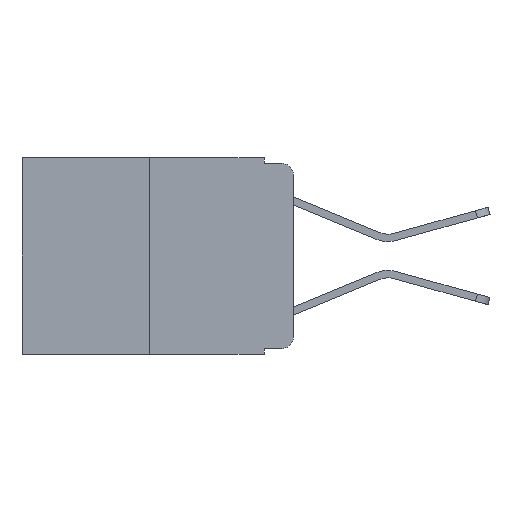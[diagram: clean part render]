
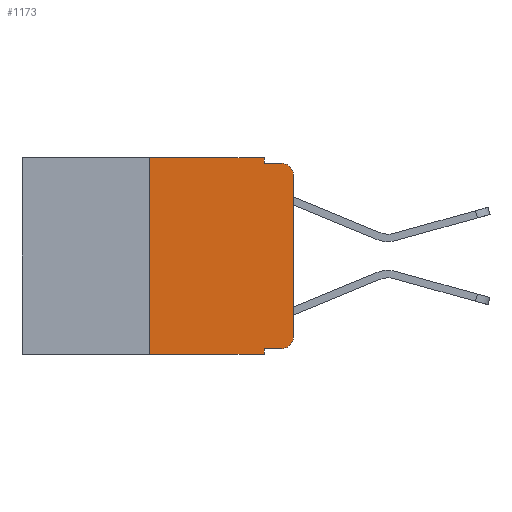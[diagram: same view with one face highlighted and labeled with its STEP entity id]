
A CAD part, left-side view. The second image highlights one B-rep face of the part: STEP entity #1173.
In plain terms, the highlighted planar face has unit normal (-1, 0, 0).
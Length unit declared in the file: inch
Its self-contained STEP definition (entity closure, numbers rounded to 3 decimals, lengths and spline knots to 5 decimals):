
#42 = DIRECTION ( 'NONE',  ( -1., 0., 0. ) ) ;
#172 = VERTEX_POINT ( 'NONE', #10972 ) ;
#308 = DIRECTION ( 'NONE',  ( 0., -1., 0. ) ) ;
#426 = EDGE_CURVE ( 'NONE', #25586, #172, #12682, .T. ) ;
#539 = CARTESIAN_POINT ( 'NONE',  ( 0., 0., -0.313 ) ) ;
#889 = DIRECTION ( 'NONE',  ( 0., 0., 1. ) ) ;
#1173 = ADVANCED_FACE ( 'NONE', ( #11707 ), #22429, .F. ) ;
#1583 = VECTOR ( 'NONE', #889, 39.37008 ) ;
#1644 = CARTESIAN_POINT ( 'NONE',  ( 0., 0.051, -0.333 ) ) ;
#1683 = VECTOR ( 'NONE', #18748, 39.37008 ) ;
#1725 = DIRECTION ( 'NONE',  ( 0., -1., 0. ) ) ;
#1880 = EDGE_CURVE ( 'NONE', #25586, #25574, #18023, .T. ) ;
#1989 = ORIENTED_EDGE ( 'NONE', *, *, #12848, .T. ) ;
#2094 = VECTOR ( 'NONE', #1725, 39.37008 ) ;
#2665 = VERTEX_POINT ( 'NONE', #5223 ) ;
#3000 = CARTESIAN_POINT ( 'NONE',  ( 0., 0.02, -0.313 ) ) ;
#3271 = EDGE_CURVE ( 'NONE', #6825, #2665, #11036, .T. ) ;
#3290 = ORIENTED_EDGE ( 'NONE', *, *, #10159, .F. ) ;
#5088 = DIRECTION ( 'NONE',  ( 0., 0., -1. ) ) ;
#5223 = CARTESIAN_POINT ( 'NONE',  ( 0., 0.25, 0. ) ) ;
#6825 = VERTEX_POINT ( 'NONE', #17806 ) ;
#7076 = VECTOR ( 'NONE', #25729, 39.37008 ) ;
#7165 = CARTESIAN_POINT ( 'NONE',  ( 0., 0.473, 0. ) ) ;
#7501 = CIRCLE ( 'NONE', #18302, 0.02 ) ;
#8603 = CARTESIAN_POINT ( 'NONE',  ( 0., 0., -0.03 ) ) ;
#8751 = ORIENTED_EDGE ( 'NONE', *, *, #16647, .F. ) ;
#9027 = VERTEX_POINT ( 'NONE', #9641 ) ;
#9124 = CARTESIAN_POINT ( 'NONE',  ( 0., 0.25, 0. ) ) ;
#9384 = EDGE_LOOP ( 'NONE', ( #11622, #1989, #24261, #3290, #8751, #14780, #20211, #15404, #26097, #10689 ) ) ;
#9475 = VECTOR ( 'NONE', #15234, 39.37008 ) ;
#9641 = CARTESIAN_POINT ( 'NONE',  ( 0., 0.051, 0. ) ) ;
#10159 = EDGE_CURVE ( 'NONE', #9027, #24816, #17827, .T. ) ;
#10689 = ORIENTED_EDGE ( 'NONE', *, *, #24200, .T. ) ;
#10972 = CARTESIAN_POINT ( 'NONE',  ( 0., 0.02, -0.333 ) ) ;
#11036 = LINE ( 'NONE', #9124, #1583 ) ;
#11107 = CARTESIAN_POINT ( 'NONE',  ( 0., 0.051, 0. ) ) ;
#11137 = CARTESIAN_POINT ( 'NONE',  ( 0., 0.051, -0.01 ) ) ;
#11517 = EDGE_CURVE ( 'NONE', #24816, #18880, #17755, .T. ) ;
#11622 = ORIENTED_EDGE ( 'NONE', *, *, #15573, .T. ) ;
#11707 = FACE_OUTER_BOUND ( 'NONE', #9384, .T. ) ;
#11789 = VECTOR ( 'NONE', #25177, 39.37008 ) ;
#12354 = DIRECTION ( 'NONE',  ( 0., -1., 0. ) ) ;
#12434 = CARTESIAN_POINT ( 'NONE',  ( 0., 0.02, -0.03 ) ) ;
#12682 = LINE ( 'NONE', #26328, #23435 ) ;
#12845 = DIRECTION ( 'NONE',  ( 1., 0., 0. ) ) ;
#12848 = EDGE_CURVE ( 'NONE', #21383, #18880, #7501, .T. ) ;
#13338 = CARTESIAN_POINT ( 'NONE',  ( 0., 0.473, 0. ) ) ;
#13634 = DIRECTION ( 'NONE',  ( 0., 0., -1. ) ) ;
#13685 = CARTESIAN_POINT ( 'NONE',  ( 0., 0., 0. ) ) ;
#14458 = DIRECTION ( 'NONE',  ( 0., 0., -1. ) ) ;
#14709 = CARTESIAN_POINT ( 'NONE',  ( 0., 0.473, -0.343 ) ) ;
#14780 = ORIENTED_EDGE ( 'NONE', *, *, #3271, .F. ) ;
#15234 = DIRECTION ( 'NONE',  ( 0., -1., 0. ) ) ;
#15404 = ORIENTED_EDGE ( 'NONE', *, *, #1880, .F. ) ;
#15573 = EDGE_CURVE ( 'NONE', #16012, #21383, #18546, .T. ) ;
#15671 = CARTESIAN_POINT ( 'NONE',  ( 0., 0.02, -0.01 ) ) ;
#15973 = CARTESIAN_POINT ( 'NONE',  ( 0., 0.051, -0.343 ) ) ;
#16012 = VERTEX_POINT ( 'NONE', #539 ) ;
#16042 = CARTESIAN_POINT ( 'NONE',  ( 0., 0.051, -0.01 ) ) ;
#16647 = EDGE_CURVE ( 'NONE', #2665, #9027, #25555, .T. ) ;
#17281 = DIRECTION ( 'NONE',  ( -1., 0., 0. ) ) ;
#17755 = LINE ( 'NONE', #16042, #2094 ) ;
#17806 = CARTESIAN_POINT ( 'NONE',  ( 0., 0.25, -0.343 ) ) ;
#17827 = LINE ( 'NONE', #11107, #11789 ) ;
#18023 = LINE ( 'NONE', #18796, #1683 ) ;
#18302 = AXIS2_PLACEMENT_3D ( 'NONE', #12434, #42, #14458 ) ;
#18546 = LINE ( 'NONE', #13685, #7076 ) ;
#18748 = DIRECTION ( 'NONE',  ( 0., 0., -1. ) ) ;
#18796 = CARTESIAN_POINT ( 'NONE',  ( 0., 0.051, 0. ) ) ;
#18880 = VERTEX_POINT ( 'NONE', #15671 ) ;
#20211 = ORIENTED_EDGE ( 'NONE', *, *, #24047, .T. ) ;
#20263 = VECTOR ( 'NONE', #308, 39.37008 ) ;
#20567 = CIRCLE ( 'NONE', #24728, 0.02 ) ;
#21383 = VERTEX_POINT ( 'NONE', #8603 ) ;
#22429 = PLANE ( 'NONE',  #24799 ) ;
#23435 = VECTOR ( 'NONE', #12354, 39.37008 ) ;
#24047 = EDGE_CURVE ( 'NONE', #6825, #25574, #24308, .T. ) ;
#24200 = EDGE_CURVE ( 'NONE', #172, #16012, #20567, .T. ) ;
#24261 = ORIENTED_EDGE ( 'NONE', *, *, #11517, .F. ) ;
#24308 = LINE ( 'NONE', #14709, #20263 ) ;
#24728 = AXIS2_PLACEMENT_3D ( 'NONE', #3000, #17281, #5088 ) ;
#24799 = AXIS2_PLACEMENT_3D ( 'NONE', #13338, #12845, #13634 ) ;
#24816 = VERTEX_POINT ( 'NONE', #11137 ) ;
#25177 = DIRECTION ( 'NONE',  ( 0., 0., -1. ) ) ;
#25555 = LINE ( 'NONE', #7165, #9475 ) ;
#25574 = VERTEX_POINT ( 'NONE', #15973 ) ;
#25586 = VERTEX_POINT ( 'NONE', #1644 ) ;
#25729 = DIRECTION ( 'NONE',  ( 0., 0., 1. ) ) ;
#26097 = ORIENTED_EDGE ( 'NONE', *, *, #426, .T. ) ;
#26328 = CARTESIAN_POINT ( 'NONE',  ( 0., 0.051, -0.333 ) ) ;
